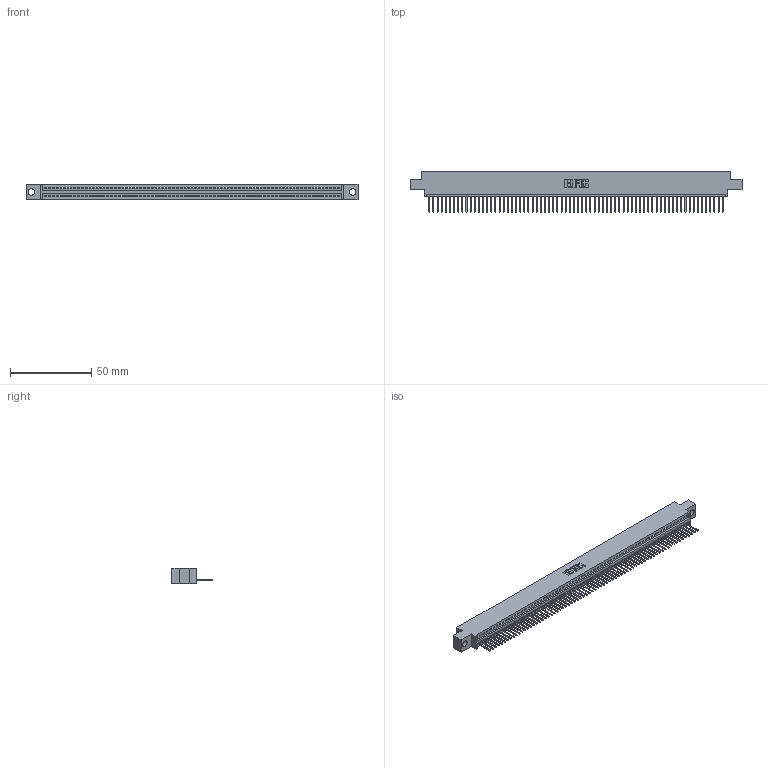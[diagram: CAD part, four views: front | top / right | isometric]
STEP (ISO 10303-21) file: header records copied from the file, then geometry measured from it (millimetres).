
FILE_DESCRIPTION (( 'STEP AP203' ), '1' );
FILE_NAME ('395-072-523-604.STEP', '2021-05-31T22:26:51', ( '' ), ( '' ), 'SwSTEP 2.0', 'SolidWorks 2020', '' );
FILE_SCHEMA (( 'CONFIG_CONTROL_DESIGN' ));
Length unit declared in the file: inch
Products named in the file (3): 345 Part_0.170 Offset - 0.156 Dia-TI; 395-072-523-604; 345-292-001_345-293-123
Assembly tree (73 placements, depth 2):
  395-072-523-604
    345 Part_0.170 Offset - 0.156 Dia-TI
    345-292-001_345-293-123  x72
Bounding box: 204.09 x 24.82 x 9.4 mm (x, y, z)
Volume: 19383.1 mm3; surface area: 26213.7 mm2
Topology: 73 solids, 73 shells, 4320 faces, 13061 edges, 8610 vertices
Faces by surface type: plane 2978, cylinder 1342
Entity records: 50719 total; most frequent: ORIENTED_EDGE 8798, CARTESIAN_POINT 8794, DIRECTION 7635, EDGE_CURVE 4399, LINE 3979, VECTOR 3979, VERTEX_POINT 2930, AXIS2_PLACEMENT_3D 1828
